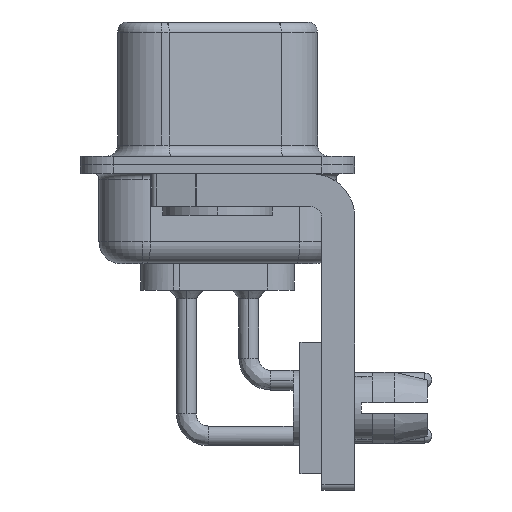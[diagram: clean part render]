
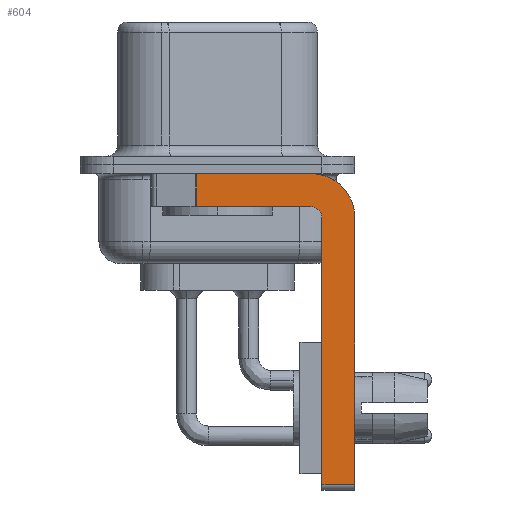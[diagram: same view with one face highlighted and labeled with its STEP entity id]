
A CAD part, left-side view. The second image highlights one B-rep face of the part: STEP entity #604.
In plain terms, the highlighted planar face has unit normal (-1, 0, 0).
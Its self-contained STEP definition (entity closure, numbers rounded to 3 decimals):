
#332 = VECTOR ( 'NONE', #35696, 1000. ) ;
#604 = ADVANCED_FACE ( 'NONE', ( #19164 ), #12399, .F. ) ;
#625 = ORIENTED_EDGE ( 'NONE', *, *, #14241, .F. ) ;
#1807 = CARTESIAN_POINT ( 'NONE',  ( -2.9, -6.25, -14.55 ) ) ;
#2099 = CARTESIAN_POINT ( 'NONE',  ( -2.9, -4.75, -14.8 ) ) ;
#2273 = EDGE_CURVE ( 'NONE', #24769, #3938, #34105, .T. ) ;
#2568 = VERTEX_POINT ( 'NONE', #3367 ) ;
#2596 = CARTESIAN_POINT ( 'NONE',  ( -2.9, 3., -0.4 ) ) ;
#3367 = CARTESIAN_POINT ( 'NONE',  ( -2.9, -4.75, -2.4 ) ) ;
#3503 = EDGE_CURVE ( 'NONE', #14116, #31247, #30577, .T. ) ;
#3568 = DIRECTION ( 'NONE',  ( 0., -1., 0. ) ) ;
#3938 = VERTEX_POINT ( 'NONE', #28208 ) ;
#4028 = DIRECTION ( 'NONE',  ( 0., 0., -1. ) ) ;
#4181 = ORIENTED_EDGE ( 'NONE', *, *, #6742, .F. ) ;
#6334 = ORIENTED_EDGE ( 'NONE', *, *, #25640, .T. ) ;
#6475 = CIRCLE ( 'NONE', #7392, 2. ) ;
#6742 = EDGE_CURVE ( 'NONE', #3938, #28266, #6475, .T. ) ;
#7121 = VECTOR ( 'NONE', #25279, 1000. ) ;
#7252 = DIRECTION ( 'NONE',  ( 1., 0., 0. ) ) ;
#7392 = AXIS2_PLACEMENT_3D ( 'NONE', #23599, #7252, #26376 ) ;
#7970 = VECTOR ( 'NONE', #32884, 1000. ) ;
#8958 = EDGE_LOOP ( 'NONE', ( #19081, #6334, #26876, #625, #9598, #13775, #15659, #4181 ) ) ;
#9598 = ORIENTED_EDGE ( 'NONE', *, *, #24287, .F. ) ;
#9703 = DIRECTION ( 'NONE',  ( -1., 0., 0. ) ) ;
#9932 = DIRECTION ( 'NONE',  ( 1., 0., 0. ) ) ;
#11667 = CARTESIAN_POINT ( 'NONE',  ( -2.9, -4.25, -14.55 ) ) ;
#12399 = PLANE ( 'NONE',  #15988 ) ;
#13775 = ORIENTED_EDGE ( 'NONE', *, *, #19018, .T. ) ;
#14116 = VERTEX_POINT ( 'NONE', #30888 ) ;
#14241 = EDGE_CURVE ( 'NONE', #2568, #14116, #29222, .T. ) ;
#14612 = LINE ( 'NONE', #34283, #29111 ) ;
#15045 = CARTESIAN_POINT ( 'NONE',  ( -2.9, 0.978, -1.9 ) ) ;
#15264 = LINE ( 'NONE', #11667, #7121 ) ;
#15659 = ORIENTED_EDGE ( 'NONE', *, *, #28632, .F. ) ;
#15988 = AXIS2_PLACEMENT_3D ( 'NONE', #30761, #9932, #18120 ) ;
#16002 = LINE ( 'NONE', #2099, #30511 ) ;
#16077 = VERTEX_POINT ( 'NONE', #18135 ) ;
#16512 = CARTESIAN_POINT ( 'NONE',  ( -2.9, -6.25, -2.4 ) ) ;
#18089 = VERTEX_POINT ( 'NONE', #1807 ) ;
#18120 = DIRECTION ( 'NONE',  ( 0., 0., -1. ) ) ;
#18135 = CARTESIAN_POINT ( 'NONE',  ( -2.9, -4.75, -14.55 ) ) ;
#19018 = EDGE_CURVE ( 'NONE', #16077, #18089, #15264, .T. ) ;
#19081 = ORIENTED_EDGE ( 'NONE', *, *, #2273, .F. ) ;
#19164 = FACE_OUTER_BOUND ( 'NONE', #8958, .T. ) ;
#19925 = CARTESIAN_POINT ( 'NONE',  ( -2.9, 0.978, -0.4 ) ) ;
#20625 = AXIS2_PLACEMENT_3D ( 'NONE', #26087, #9703, #28801 ) ;
#21424 = DIRECTION ( 'NONE',  ( 0., 0., 1. ) ) ;
#23599 = CARTESIAN_POINT ( 'NONE',  ( -2.9, -4.25, -2.4 ) ) ;
#24287 = EDGE_CURVE ( 'NONE', #16077, #2568, #16002, .T. ) ;
#24769 = VERTEX_POINT ( 'NONE', #19925 ) ;
#25279 = DIRECTION ( 'NONE',  ( 0., -1., 0. ) ) ;
#25640 = EDGE_CURVE ( 'NONE', #24769, #31247, #14612, .T. ) ;
#26087 = CARTESIAN_POINT ( 'NONE',  ( -2.9, -4.25, -2.4 ) ) ;
#26376 = DIRECTION ( 'NONE',  ( 0., 0., -1. ) ) ;
#26876 = ORIENTED_EDGE ( 'NONE', *, *, #3503, .F. ) ;
#28208 = CARTESIAN_POINT ( 'NONE',  ( -2.9, -4.25, -0.4 ) ) ;
#28266 = VERTEX_POINT ( 'NONE', #34111 ) ;
#28632 = EDGE_CURVE ( 'NONE', #28266, #18089, #35384, .T. ) ;
#28801 = DIRECTION ( 'NONE',  ( 0., 0., 1. ) ) ;
#29111 = VECTOR ( 'NONE', #4028, 1000. ) ;
#29222 = CIRCLE ( 'NONE', #20625, 0.5 ) ;
#30511 = VECTOR ( 'NONE', #21424, 1000. ) ;
#30577 = LINE ( 'NONE', #35606, #332 ) ;
#30761 = CARTESIAN_POINT ( 'NONE',  ( -2.9, -4.25, -2.4 ) ) ;
#30888 = CARTESIAN_POINT ( 'NONE',  ( -2.9, -4.25, -1.9 ) ) ;
#31247 = VERTEX_POINT ( 'NONE', #15045 ) ;
#32884 = DIRECTION ( 'NONE',  ( 0., 0., -1. ) ) ;
#33233 = VECTOR ( 'NONE', #3568, 1000. ) ;
#34105 = LINE ( 'NONE', #2596, #33233 ) ;
#34111 = CARTESIAN_POINT ( 'NONE',  ( -2.9, -6.25, -2.4 ) ) ;
#34283 = CARTESIAN_POINT ( 'NONE',  ( -2.9, 0.978, -1.9 ) ) ;
#35384 = LINE ( 'NONE', #16512, #7970 ) ;
#35606 = CARTESIAN_POINT ( 'NONE',  ( -2.9, -4.25, -1.9 ) ) ;
#35696 = DIRECTION ( 'NONE',  ( 0., 1., 0. ) ) ;
